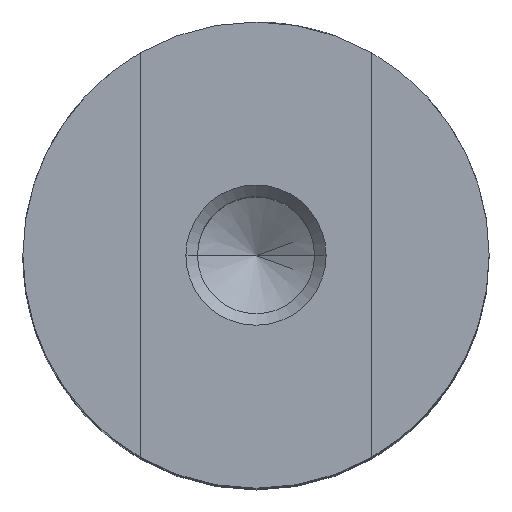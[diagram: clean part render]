
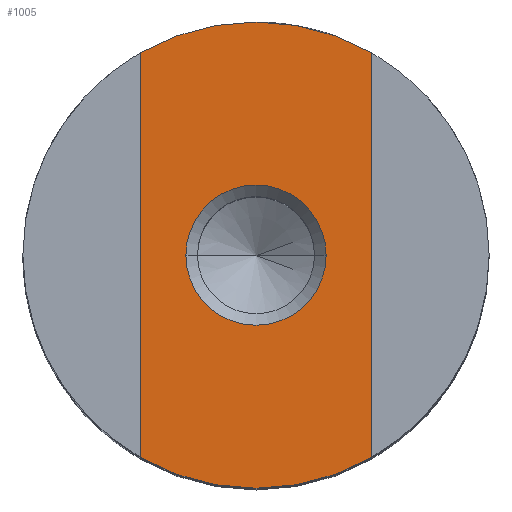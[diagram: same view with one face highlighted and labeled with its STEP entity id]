
A CAD part, top view. The second image highlights one B-rep face of the part: STEP entity #1005.
In plain terms, the highlighted planar face has unit normal (0, 0, 1).
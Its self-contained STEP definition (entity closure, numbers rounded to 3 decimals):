
#11 = FACE_OUTER_BOUND ( 'NONE', #1133, .T. ) ;
#13 = AXIS2_PLACEMENT_3D ( 'NONE', #30, #28, #25 ) ;
#16 = FACE_BOUND ( 'NONE', #1079, .T. ) ;
#25 = DIRECTION ( 'NONE',  ( 1., 0., 0. ) ) ;
#26 = DIRECTION ( 'NONE',  ( 1., 0., 0. ) ) ;
#28 = DIRECTION ( 'NONE',  ( 0., 0., 1. ) ) ;
#30 = CARTESIAN_POINT ( 'NONE',  ( 0., 0., -1.63 ) ) ;
#72 = CARTESIAN_POINT ( 'NONE',  ( -1.422, 0., -1.63 ) ) ;
#104 = VECTOR ( 'NONE', #171, 1000. ) ;
#106 = LINE ( 'NONE', #477, #104 ) ;
#113 = VECTOR ( 'NONE', #623, 1000. ) ;
#122 = LINE ( 'NONE', #778, #113 ) ;
#144 = CIRCLE ( 'NONE', #1368, 1.422 ) ;
#171 = DIRECTION ( 'NONE',  ( 0., 1., 0. ) ) ;
#187 = CIRCLE ( 'NONE', #800, 4.73 ) ;
#218 = DIRECTION ( 'NONE',  ( 0., 0., -1. ) ) ;
#227 = PLANE ( 'NONE',  #1393 ) ;
#232 = AXIS2_PLACEMENT_3D ( 'NONE', #561, #1458, #380 ) ;
#245 = EDGE_CURVE ( 'NONE', #1049, #1073, #502, .T. ) ;
#316 = CARTESIAN_POINT ( 'NONE',  ( 2.35, 4.105, -1.63 ) ) ;
#369 = EDGE_CURVE ( 'NONE', #762, #772, #395, .T. ) ;
#379 = DIRECTION ( 'NONE',  ( -1., 0., 0. ) ) ;
#380 = DIRECTION ( 'NONE',  ( -1., 0., 0. ) ) ;
#395 = CIRCLE ( 'NONE', #232, 4.73 ) ;
#477 = CARTESIAN_POINT ( 'NONE',  ( 2.35, -4.73, -1.63 ) ) ;
#502 = CIRCLE ( 'NONE', #13, 1.422 ) ;
#561 = CARTESIAN_POINT ( 'NONE',  ( 0., 0., -1.63 ) ) ;
#563 = DIRECTION ( 'NONE',  ( -1., 0., 0. ) ) ;
#623 = DIRECTION ( 'NONE',  ( 0., 1., 0. ) ) ;
#712 = EDGE_CURVE ( 'NONE', #926, #979, #187, .T. ) ;
#762 = VERTEX_POINT ( 'NONE', #1120 ) ;
#772 = VERTEX_POINT ( 'NONE', #316 ) ;
#778 = CARTESIAN_POINT ( 'NONE',  ( -2.35, -4.73, -1.63 ) ) ;
#780 = EDGE_CURVE ( 'NONE', #1073, #1049, #144, .T. ) ;
#784 = EDGE_CURVE ( 'NONE', #979, #762, #122, .T. ) ;
#794 = EDGE_CURVE ( 'NONE', #926, #772, #106, .T. ) ;
#800 = AXIS2_PLACEMENT_3D ( 'NONE', #995, #933, #563 ) ;
#843 = CARTESIAN_POINT ( 'NONE',  ( 1.422, 0., -1.63 ) ) ;
#910 = DIRECTION ( 'NONE',  ( 0., 0., 1. ) ) ;
#926 = VERTEX_POINT ( 'NONE', #1047 ) ;
#933 = DIRECTION ( 'NONE',  ( 0., 0., -1. ) ) ;
#953 = CARTESIAN_POINT ( 'NONE',  ( -2.35, -4.73, -1.63 ) ) ;
#979 = VERTEX_POINT ( 'NONE', #1058 ) ;
#995 = CARTESIAN_POINT ( 'NONE',  ( 0., 0., -1.63 ) ) ;
#1005 = ADVANCED_FACE ( 'NONE', ( #16, #11 ), #227, .F. ) ;
#1047 = CARTESIAN_POINT ( 'NONE',  ( 2.35, -4.105, -1.63 ) ) ;
#1049 = VERTEX_POINT ( 'NONE', #72 ) ;
#1058 = CARTESIAN_POINT ( 'NONE',  ( -2.35, -4.105, -1.63 ) ) ;
#1073 = VERTEX_POINT ( 'NONE', #843 ) ;
#1079 = EDGE_LOOP ( 'NONE', ( #1240, #1269 ) ) ;
#1120 = CARTESIAN_POINT ( 'NONE',  ( -2.35, 4.105, -1.63 ) ) ;
#1133 = EDGE_LOOP ( 'NONE', ( #1332, #1289, #1295, #1306 ) ) ;
#1240 = ORIENTED_EDGE ( 'NONE', *, *, #780, .F. ) ;
#1269 = ORIENTED_EDGE ( 'NONE', *, *, #245, .F. ) ;
#1289 = ORIENTED_EDGE ( 'NONE', *, *, #712, .F. ) ;
#1295 = ORIENTED_EDGE ( 'NONE', *, *, #794, .T. ) ;
#1306 = ORIENTED_EDGE ( 'NONE', *, *, #369, .F. ) ;
#1332 = ORIENTED_EDGE ( 'NONE', *, *, #784, .F. ) ;
#1368 = AXIS2_PLACEMENT_3D ( 'NONE', #1454, #910, #26 ) ;
#1393 = AXIS2_PLACEMENT_3D ( 'NONE', #953, #218, #379 ) ;
#1454 = CARTESIAN_POINT ( 'NONE',  ( 0., 0., -1.63 ) ) ;
#1458 = DIRECTION ( 'NONE',  ( 0., 0., -1. ) ) ;
